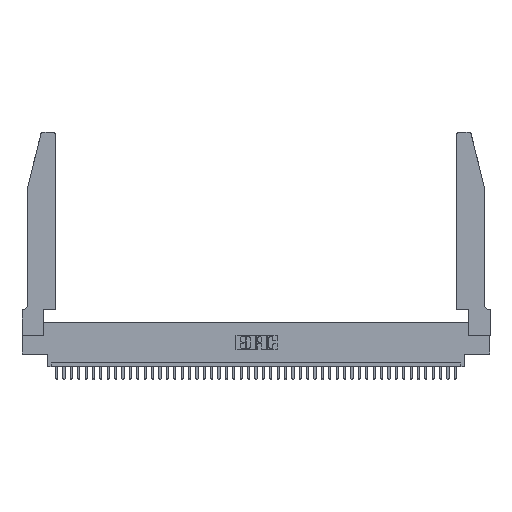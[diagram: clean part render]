
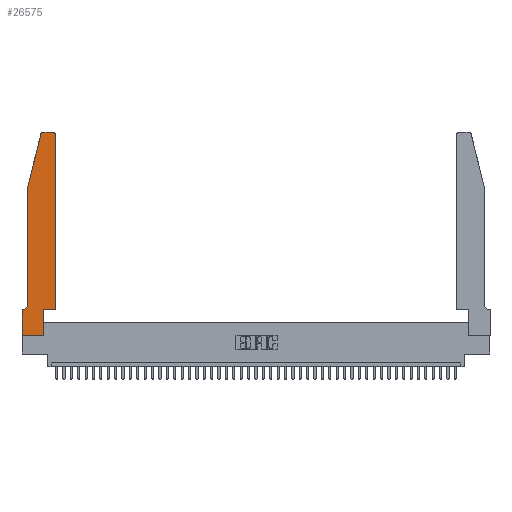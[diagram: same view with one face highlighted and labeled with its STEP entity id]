
A CAD part, top view. The second image highlights one B-rep face of the part: STEP entity #26575.
In plain terms, the highlighted planar face has unit normal (0, 0, 1).
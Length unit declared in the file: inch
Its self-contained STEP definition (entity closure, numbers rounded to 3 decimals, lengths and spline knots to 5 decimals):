
#453 = DIRECTION ( 'NONE',  ( 0., -1., 0. ) ) ;
#682 = CARTESIAN_POINT ( 'NONE',  ( 0.4505, 0.35, 0.37 ) ) ;
#694 = CARTESIAN_POINT ( 'NONE',  ( 0., 0., 0.37 ) ) ;
#998 = DIRECTION ( 'NONE',  ( 0., 0., 1. ) ) ;
#1221 = LINE ( 'NONE', #34172, #31996 ) ;
#1452 = LINE ( 'NONE', #26310, #12766 ) ;
#2079 = LINE ( 'NONE', #41733, #17137 ) ;
#3791 = EDGE_CURVE ( 'NONE', #27032, #24875, #34006, .T. ) ;
#3805 = CARTESIAN_POINT ( 'NONE',  ( 0.4505, 0.35, 0.37 ) ) ;
#4262 = AXIS2_PLACEMENT_3D ( 'NONE', #16199, #16492, #40468 ) ;
#4635 = AXIS2_PLACEMENT_3D ( 'NONE', #21459, #998, #35225 ) ;
#5452 = VECTOR ( 'NONE', #27009, 39.37008 ) ;
#5841 = DIRECTION ( 'NONE',  ( -0.239, -0.971, 0. ) ) ;
#6378 = VECTOR ( 'NONE', #5841, 39.37008 ) ;
#6722 = EDGE_LOOP ( 'NONE', ( #28300, #7647, #40454, #14068, #16671, #15899, #22940, #40593, #30190, #11402, #42233, #32491 ) ) ;
#7311 = EDGE_CURVE ( 'NONE', #38465, #35279, #17707, .T. ) ;
#7647 = ORIENTED_EDGE ( 'NONE', *, *, #43782, .T. ) ;
#7728 = CARTESIAN_POINT ( 'NONE',  ( 0.25487, 2.72718, 0.37 ) ) ;
#8648 = LINE ( 'NONE', #9588, #14565 ) ;
#9588 = CARTESIAN_POINT ( 'NONE',  ( 0.2605, 2.75, 0.37 ) ) ;
#9649 = VERTEX_POINT ( 'NONE', #15970 ) ;
#10472 = CARTESIAN_POINT ( 'NONE',  ( 0.0755, 0.42, 0.37 ) ) ;
#11262 = DIRECTION ( 'NONE',  ( 1., 0., 0. ) ) ;
#11402 = ORIENTED_EDGE ( 'NONE', *, *, #20100, .T. ) ;
#11502 = EDGE_CURVE ( 'NONE', #39809, #23051, #43817, .T. ) ;
#12447 = CIRCLE ( 'NONE', #14102, 0.07 ) ;
#12766 = VECTOR ( 'NONE', #40606, 39.37008 ) ;
#13295 = FACE_OUTER_BOUND ( 'NONE', #6722, .T. ) ;
#14068 = ORIENTED_EDGE ( 'NONE', *, *, #14347, .T. ) ;
#14102 = AXIS2_PLACEMENT_3D ( 'NONE', #18754, #42583, #28896 ) ;
#14347 = EDGE_CURVE ( 'NONE', #35279, #24211, #2079, .T. ) ;
#14371 = CARTESIAN_POINT ( 'NONE',  ( 0.2865, 0.35, 0.37 ) ) ;
#14503 = LINE ( 'NONE', #33225, #24751 ) ;
#14557 = VECTOR ( 'NONE', #27923, 39.37008 ) ;
#14565 = VECTOR ( 'NONE', #17080, 39.37008 ) ;
#14668 = EDGE_CURVE ( 'NONE', #24875, #42751, #24689, .T. ) ;
#14887 = CARTESIAN_POINT ( 'NONE',  ( 0.2865, 0., 0.37 ) ) ;
#15899 = ORIENTED_EDGE ( 'NONE', *, *, #41299, .T. ) ;
#15970 = CARTESIAN_POINT ( 'NONE',  ( 0.284, 2.75, 0.37 ) ) ;
#16199 = CARTESIAN_POINT ( 'NONE',  ( 0.4205, 2.72, 0.37 ) ) ;
#16492 = DIRECTION ( 'NONE',  ( 0., 0., 1. ) ) ;
#16671 = ORIENTED_EDGE ( 'NONE', *, *, #29132, .T. ) ;
#16721 = CARTESIAN_POINT ( 'NONE',  ( 0.0755, 0.35, 0.37 ) ) ;
#17080 = DIRECTION ( 'NONE',  ( -1., 0., 0. ) ) ;
#17137 = VECTOR ( 'NONE', #453, 39.37008 ) ;
#17245 = DIRECTION ( 'NONE',  ( 0., -1., 0. ) ) ;
#17707 = LINE ( 'NONE', #22993, #6378 ) ;
#18754 = CARTESIAN_POINT ( 'NONE',  ( 0.0055, 0.42, 0.37 ) ) ;
#19040 = VERTEX_POINT ( 'NONE', #27419 ) ;
#19914 = CARTESIAN_POINT ( 'NONE',  ( 0., 0.35, 0.37 ) ) ;
#20100 = EDGE_CURVE ( 'NONE', #32873, #27032, #14503, .T. ) ;
#21459 = CARTESIAN_POINT ( 'NONE',  ( 0.284, 2.72, 0.37 ) ) ;
#21785 = DIRECTION ( 'NONE',  ( 0., 0., 1. ) ) ;
#22071 = DIRECTION ( 'NONE',  ( 1., 0., 0. ) ) ;
#22767 = DIRECTION ( 'NONE',  ( 1., 0., 0. ) ) ;
#22940 = ORIENTED_EDGE ( 'NONE', *, *, #40709, .T. ) ;
#22993 = CARTESIAN_POINT ( 'NONE',  ( 0.0755, 2., 0.37 ) ) ;
#23051 = VERTEX_POINT ( 'NONE', #14887 ) ;
#23775 = CARTESIAN_POINT ( 'NONE',  ( 0., 0., 0.37 ) ) ;
#24211 = VERTEX_POINT ( 'NONE', #10472 ) ;
#24689 = CIRCLE ( 'NONE', #4262, 0.03 ) ;
#24751 = VECTOR ( 'NONE', #22767, 39.37008 ) ;
#24875 = VERTEX_POINT ( 'NONE', #39861 ) ;
#25401 = PLANE ( 'NONE',  #32534 ) ;
#26310 = CARTESIAN_POINT ( 'NONE',  ( 0.2865, 0.35, 0.37 ) ) ;
#26502 = LINE ( 'NONE', #16721, #5452 ) ;
#26575 = ADVANCED_FACE ( 'NONE', ( #13295 ), #25401, .T. ) ;
#27009 = DIRECTION ( 'NONE',  ( -1., 0., 0. ) ) ;
#27032 = VERTEX_POINT ( 'NONE', #682 ) ;
#27419 = CARTESIAN_POINT ( 'NONE',  ( 0.0055, 0.35, 0.37 ) ) ;
#27923 = DIRECTION ( 'NONE',  ( 0., 1., 0. ) ) ;
#28300 = ORIENTED_EDGE ( 'NONE', *, *, #29359, .T. ) ;
#28674 = CARTESIAN_POINT ( 'NONE',  ( 0.4205, 2.75, 0.37 ) ) ;
#28896 = DIRECTION ( 'NONE',  ( -1., 0., 0. ) ) ;
#29132 = EDGE_CURVE ( 'NONE', #24211, #19040, #12447, .T. ) ;
#29359 = EDGE_CURVE ( 'NONE', #42751, #9649, #8648, .T. ) ;
#30190 = ORIENTED_EDGE ( 'NONE', *, *, #37737, .T. ) ;
#31996 = VECTOR ( 'NONE', #17245, 39.37008 ) ;
#32491 = ORIENTED_EDGE ( 'NONE', *, *, #14668, .T. ) ;
#32534 = AXIS2_PLACEMENT_3D ( 'NONE', #35405, #21785, #22071 ) ;
#32637 = VERTEX_POINT ( 'NONE', #19914 ) ;
#32873 = VERTEX_POINT ( 'NONE', #14371 ) ;
#33225 = CARTESIAN_POINT ( 'NONE',  ( 0.4505, 0.35, 0.37 ) ) ;
#34006 = LINE ( 'NONE', #3805, #14557 ) ;
#34172 = CARTESIAN_POINT ( 'NONE',  ( 0., 0., 0.37 ) ) ;
#35225 = DIRECTION ( 'NONE',  ( 1., 0., 0. ) ) ;
#35279 = VERTEX_POINT ( 'NONE', #37062 ) ;
#35405 = CARTESIAN_POINT ( 'NONE',  ( 0., 0.35, 0.37 ) ) ;
#37062 = CARTESIAN_POINT ( 'NONE',  ( 0.0755, 2., 0.37 ) ) ;
#37737 = EDGE_CURVE ( 'NONE', #23051, #32873, #1452, .T. ) ;
#38465 = VERTEX_POINT ( 'NONE', #7728 ) ;
#39809 = VERTEX_POINT ( 'NONE', #23775 ) ;
#39861 = CARTESIAN_POINT ( 'NONE',  ( 0.4505, 2.72, 0.37 ) ) ;
#40454 = ORIENTED_EDGE ( 'NONE', *, *, #7311, .T. ) ;
#40468 = DIRECTION ( 'NONE',  ( 1., 0., 0. ) ) ;
#40562 = VECTOR ( 'NONE', #11262, 39.37008 ) ;
#40593 = ORIENTED_EDGE ( 'NONE', *, *, #11502, .T. ) ;
#40606 = DIRECTION ( 'NONE',  ( 0., 1., 0. ) ) ;
#40709 = EDGE_CURVE ( 'NONE', #32637, #39809, #1221, .T. ) ;
#41290 = CIRCLE ( 'NONE', #4635, 0.03 ) ;
#41299 = EDGE_CURVE ( 'NONE', #19040, #32637, #26502, .T. ) ;
#41733 = CARTESIAN_POINT ( 'NONE',  ( 0.0755, 2., 0.37 ) ) ;
#42233 = ORIENTED_EDGE ( 'NONE', *, *, #3791, .T. ) ;
#42583 = DIRECTION ( 'NONE',  ( 0., 0., -1. ) ) ;
#42751 = VERTEX_POINT ( 'NONE', #28674 ) ;
#43782 = EDGE_CURVE ( 'NONE', #9649, #38465, #41290, .T. ) ;
#43817 = LINE ( 'NONE', #694, #40562 ) ;
